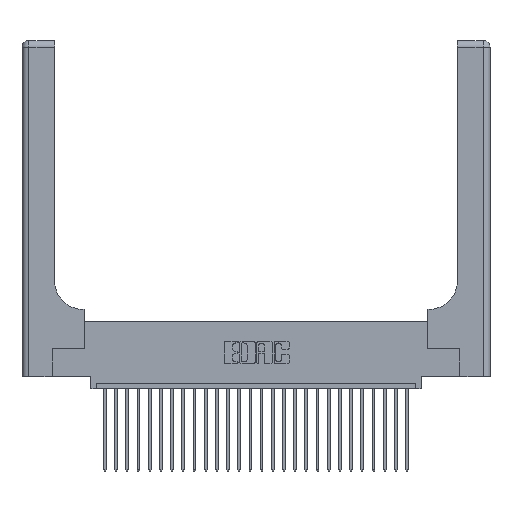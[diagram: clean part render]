
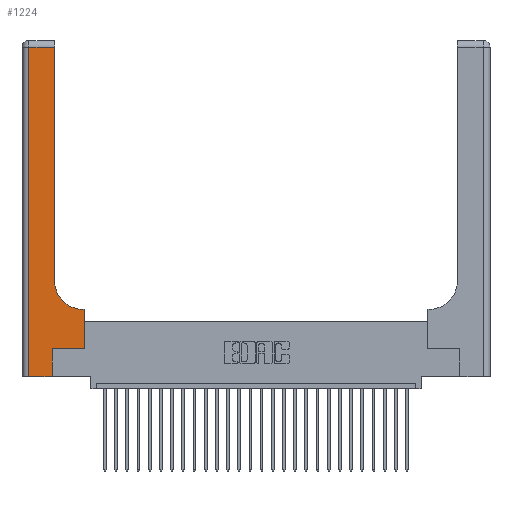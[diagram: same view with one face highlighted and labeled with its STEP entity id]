
A CAD part, top view. The second image highlights one B-rep face of the part: STEP entity #1224.
In plain terms, the highlighted planar face has unit normal (0, 0, 1).
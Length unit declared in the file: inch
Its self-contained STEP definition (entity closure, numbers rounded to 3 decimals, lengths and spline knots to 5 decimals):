
#705 = CARTESIAN_POINT ( 'NONE',  ( 0.269, 0., 0.37 ) ) ;
#1224 = ADVANCED_FACE ( 'NONE', ( #19742 ), #6091, .F. ) ;
#1902 = VERTEX_POINT ( 'NONE', #3901 ) ;
#2111 = VERTEX_POINT ( 'NONE', #3935 ) ;
#2238 = ORIENTED_EDGE ( 'NONE', *, *, #17945, .T. ) ;
#2661 = VECTOR ( 'NONE', #27716, 39.37008 ) ;
#3575 = LINE ( 'NONE', #4335, #21076 ) ;
#3857 = LINE ( 'NONE', #9786, #8635 ) ;
#3901 = CARTESIAN_POINT ( 'NONE',  ( 0.06, 0., 0.37 ) ) ;
#3911 = LINE ( 'NONE', #25376, #14890 ) ;
#3935 = CARTESIAN_POINT ( 'NONE',  ( 0.06, 2.94, 0.37 ) ) ;
#4335 = CARTESIAN_POINT ( 'NONE',  ( 0.269, 0., 0.37 ) ) ;
#4486 = CARTESIAN_POINT ( 'NONE',  ( 0.5585, 0.25, 0.37 ) ) ;
#5176 = ORIENTED_EDGE ( 'NONE', *, *, #15926, .T. ) ;
#5285 = DIRECTION ( 'NONE',  ( 0., 0., -1. ) ) ;
#5720 = ORIENTED_EDGE ( 'NONE', *, *, #6261, .T. ) ;
#6091 = PLANE ( 'NONE',  #7187 ) ;
#6261 = EDGE_CURVE ( 'NONE', #1902, #20162, #7740, .T. ) ;
#6386 = EDGE_CURVE ( 'NONE', #25787, #14885, #27551, .T. ) ;
#7040 = VECTOR ( 'NONE', #20299, 39.37008 ) ;
#7187 = AXIS2_PLACEMENT_3D ( 'NONE', #19255, #27930, #17700 ) ;
#7300 = DIRECTION ( 'NONE',  ( 1., 0., 0. ) ) ;
#7740 = LINE ( 'NONE', #11252, #7040 ) ;
#8635 = VECTOR ( 'NONE', #11838, 39.37008 ) ;
#8862 = ORIENTED_EDGE ( 'NONE', *, *, #6386, .T. ) ;
#9581 = VERTEX_POINT ( 'NONE', #18233 ) ;
#9612 = LINE ( 'NONE', #14104, #15787 ) ;
#9786 = CARTESIAN_POINT ( 'NONE',  ( 0., 2.94, 0.37 ) ) ;
#10057 = VECTOR ( 'NONE', #20707, 39.37008 ) ;
#10413 = EDGE_CURVE ( 'NONE', #2111, #1902, #9612, .T. ) ;
#11252 = CARTESIAN_POINT ( 'NONE',  ( 0., 0., 0.37 ) ) ;
#11720 = ORIENTED_EDGE ( 'NONE', *, *, #21453, .T. ) ;
#11838 = DIRECTION ( 'NONE',  ( -1., 0., 0. ) ) ;
#12669 = LINE ( 'NONE', #18843, #2661 ) ;
#13194 = ORIENTED_EDGE ( 'NONE', *, *, #10413, .T. ) ;
#13352 = AXIS2_PLACEMENT_3D ( 'NONE', #18440, #5285, #7300 ) ;
#14104 = CARTESIAN_POINT ( 'NONE',  ( 0.06, 3., 0.37 ) ) ;
#14360 = ORIENTED_EDGE ( 'NONE', *, *, #19468, .T. ) ;
#14885 = VERTEX_POINT ( 'NONE', #25991 ) ;
#14890 = VECTOR ( 'NONE', #16730, 39.37008 ) ;
#15621 = ORIENTED_EDGE ( 'NONE', *, *, #18166, .T. ) ;
#15787 = VECTOR ( 'NONE', #27382, 39.37008 ) ;
#15813 = ORIENTED_EDGE ( 'NONE', *, *, #18299, .T. ) ;
#15926 = EDGE_CURVE ( 'NONE', #14885, #9581, #17711, .T. ) ;
#16730 = DIRECTION ( 'NONE',  ( -1., 0., 0. ) ) ;
#17270 = VERTEX_POINT ( 'NONE', #4486 ) ;
#17679 = DIRECTION ( 'NONE',  ( 0., 1., 0. ) ) ;
#17700 = DIRECTION ( 'NONE',  ( -1., 0., 0. ) ) ;
#17711 = LINE ( 'NONE', #28026, #26515 ) ;
#17937 = LINE ( 'NONE', #21093, #10057 ) ;
#17945 = EDGE_CURVE ( 'NONE', #17270, #19161, #17937, .T. ) ;
#18166 = EDGE_CURVE ( 'NONE', #19161, #25787, #3911, .T. ) ;
#18233 = CARTESIAN_POINT ( 'NONE',  ( 0.2915, 2.94, 0.37 ) ) ;
#18299 = EDGE_CURVE ( 'NONE', #20162, #26267, #3575, .T. ) ;
#18440 = CARTESIAN_POINT ( 'NONE',  ( 0.5415, 0.85, 0.37 ) ) ;
#18843 = CARTESIAN_POINT ( 'NONE',  ( 0.269, 0.25, 0.37 ) ) ;
#19161 = VERTEX_POINT ( 'NONE', #24215 ) ;
#19255 = CARTESIAN_POINT ( 'NONE',  ( 0., 3., 0.37 ) ) ;
#19468 = EDGE_CURVE ( 'NONE', #9581, #2111, #3857, .T. ) ;
#19742 = FACE_OUTER_BOUND ( 'NONE', #23178, .T. ) ;
#20130 = CARTESIAN_POINT ( 'NONE',  ( 0.5415, 0.6, 0.37 ) ) ;
#20162 = VERTEX_POINT ( 'NONE', #705 ) ;
#20299 = DIRECTION ( 'NONE',  ( 1., 0., 0. ) ) ;
#20707 = DIRECTION ( 'NONE',  ( 0., 1., 0. ) ) ;
#21076 = VECTOR ( 'NONE', #17679, 39.37008 ) ;
#21093 = CARTESIAN_POINT ( 'NONE',  ( 0.5585, 0.25, 0.37 ) ) ;
#21189 = DIRECTION ( 'NONE',  ( 0., 1., 0. ) ) ;
#21453 = EDGE_CURVE ( 'NONE', #26267, #17270, #12669, .T. ) ;
#23178 = EDGE_LOOP ( 'NONE', ( #5176, #14360, #13194, #5720, #15813, #11720, #2238, #15621, #8862 ) ) ;
#24215 = CARTESIAN_POINT ( 'NONE',  ( 0.5585, 0.6, 0.37 ) ) ;
#25376 = CARTESIAN_POINT ( 'NONE',  ( 0.2915, 0.6, 0.37 ) ) ;
#25787 = VERTEX_POINT ( 'NONE', #20130 ) ;
#25991 = CARTESIAN_POINT ( 'NONE',  ( 0.2915, 0.85, 0.37 ) ) ;
#26267 = VERTEX_POINT ( 'NONE', #26654 ) ;
#26515 = VECTOR ( 'NONE', #21189, 39.37008 ) ;
#26654 = CARTESIAN_POINT ( 'NONE',  ( 0.269, 0.25, 0.37 ) ) ;
#27382 = DIRECTION ( 'NONE',  ( 0., -1., 0. ) ) ;
#27551 = CIRCLE ( 'NONE', #13352, 0.25 ) ;
#27716 = DIRECTION ( 'NONE',  ( 1., 0., 0. ) ) ;
#27930 = DIRECTION ( 'NONE',  ( 0., 0., -1. ) ) ;
#28026 = CARTESIAN_POINT ( 'NONE',  ( 0.2915, 3., 0.37 ) ) ;
